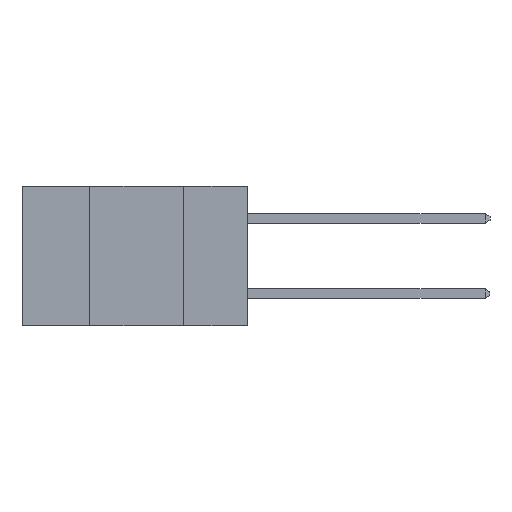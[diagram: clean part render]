
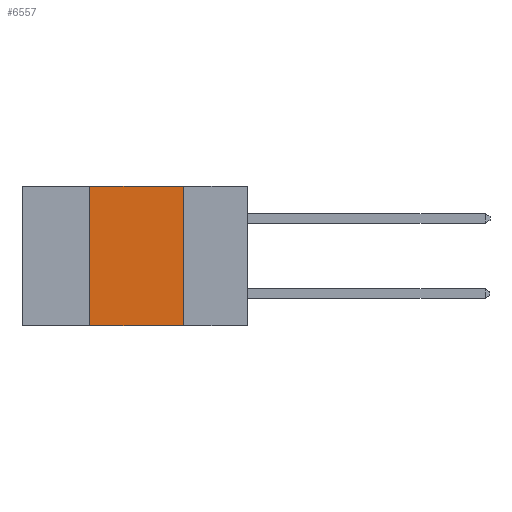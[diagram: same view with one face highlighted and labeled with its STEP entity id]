
A CAD part, left-side view. The second image highlights one B-rep face of the part: STEP entity #6557.
In plain terms, the highlighted planar face has unit normal (-1, 0, 0).
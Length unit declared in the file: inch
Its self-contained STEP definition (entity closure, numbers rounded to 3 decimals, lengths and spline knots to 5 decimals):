
#390 = CARTESIAN_POINT ( 'NONE',  ( 0., 0.6, 0. ) ) ;
#599 = CARTESIAN_POINT ( 'NONE',  ( 0., 0.6, 0. ) ) ;
#1271 = CARTESIAN_POINT ( 'NONE',  ( 0., 0.42, -0.37 ) ) ;
#1750 = LINE ( 'NONE', #8035, #15031 ) ;
#2574 = VERTEX_POINT ( 'NONE', #1271 ) ;
#3078 = LINE ( 'NONE', #14322, #6184 ) ;
#3316 = DIRECTION ( 'NONE',  ( 0., 0., -1. ) ) ;
#3655 = DIRECTION ( 'NONE',  ( 0., -1., 0. ) ) ;
#3905 = CARTESIAN_POINT ( 'NONE',  ( 0., 0.17, 0. ) ) ;
#4325 = LINE ( 'NONE', #3905, #14540 ) ;
#4371 = ORIENTED_EDGE ( 'NONE', *, *, #9357, .F. ) ;
#4429 = DIRECTION ( 'NONE',  ( 0., -1., 0. ) ) ;
#4646 = DIRECTION ( 'NONE',  ( 0., 0., 1. ) ) ;
#4660 = EDGE_LOOP ( 'NONE', ( #5604, #4371, #14966, #5234 ) ) ;
#4840 = EDGE_CURVE ( 'NONE', #2574, #15809, #1750, .T. ) ;
#5234 = ORIENTED_EDGE ( 'NONE', *, *, #8451, .T. ) ;
#5604 = ORIENTED_EDGE ( 'NONE', *, *, #7899, .F. ) ;
#6184 = VECTOR ( 'NONE', #3655, 39.37008 ) ;
#6557 = ADVANCED_FACE ( 'NONE', ( #11545 ), #9995, .F. ) ;
#7899 = EDGE_CURVE ( 'NONE', #13269, #11664, #4325, .T. ) ;
#8035 = CARTESIAN_POINT ( 'NONE',  ( 0., 0.42, 0. ) ) ;
#8451 = EDGE_CURVE ( 'NONE', #2574, #11664, #3078, .T. ) ;
#8993 = CARTESIAN_POINT ( 'NONE',  ( 0., 0.42, 0. ) ) ;
#9357 = EDGE_CURVE ( 'NONE', #15809, #13269, #16081, .T. ) ;
#9995 = PLANE ( 'NONE',  #14785 ) ;
#10562 = DIRECTION ( 'NONE',  ( 0., 0., -1. ) ) ;
#11360 = DIRECTION ( 'NONE',  ( 1., 0., 0. ) ) ;
#11480 = CARTESIAN_POINT ( 'NONE',  ( 0., 0.17, 0. ) ) ;
#11545 = FACE_OUTER_BOUND ( 'NONE', #4660, .T. ) ;
#11664 = VERTEX_POINT ( 'NONE', #13768 ) ;
#12701 = VECTOR ( 'NONE', #4429, 39.37008 ) ;
#13269 = VERTEX_POINT ( 'NONE', #11480 ) ;
#13768 = CARTESIAN_POINT ( 'NONE',  ( 0., 0.17, -0.37 ) ) ;
#14322 = CARTESIAN_POINT ( 'NONE',  ( 0., 0.6, -0.37 ) ) ;
#14540 = VECTOR ( 'NONE', #10562, 39.37008 ) ;
#14785 = AXIS2_PLACEMENT_3D ( 'NONE', #599, #11360, #3316 ) ;
#14966 = ORIENTED_EDGE ( 'NONE', *, *, #4840, .F. ) ;
#15031 = VECTOR ( 'NONE', #4646, 39.37008 ) ;
#15809 = VERTEX_POINT ( 'NONE', #8993 ) ;
#16081 = LINE ( 'NONE', #390, #12701 ) ;
